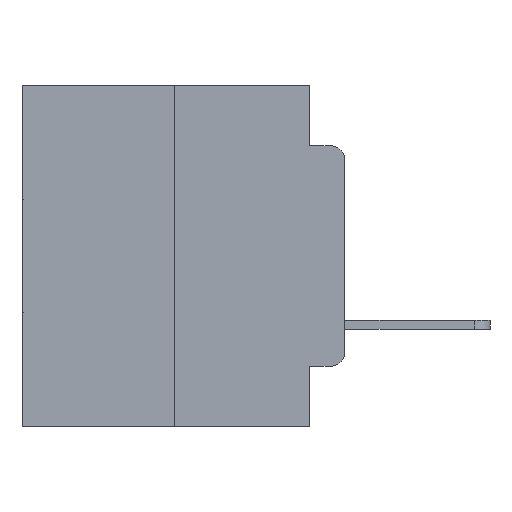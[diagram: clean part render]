
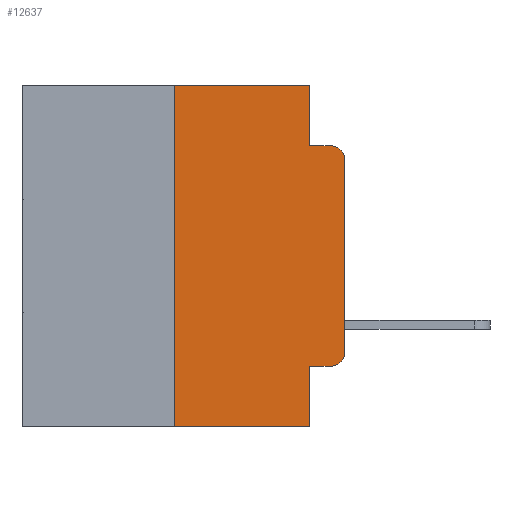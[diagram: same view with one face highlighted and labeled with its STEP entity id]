
A CAD part, left-side view. The second image highlights one B-rep face of the part: STEP entity #12637.
In plain terms, the highlighted planar face has unit normal (-1, 0, 0).
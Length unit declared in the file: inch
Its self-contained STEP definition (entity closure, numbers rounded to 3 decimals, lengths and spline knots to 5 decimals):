
#293 = CARTESIAN_POINT ( 'NONE',  ( 0., 0.473, 0. ) ) ;
#417 = ORIENTED_EDGE ( 'NONE', *, *, #3928, .F. ) ;
#593 = ORIENTED_EDGE ( 'NONE', *, *, #23542, .F. ) ;
#692 = EDGE_CURVE ( 'NONE', #3797, #19112, #18793, .T. ) ;
#924 = ORIENTED_EDGE ( 'NONE', *, *, #692, .F. ) ;
#1023 = ORIENTED_EDGE ( 'NONE', *, *, #10086, .T. ) ;
#1326 = CARTESIAN_POINT ( 'NONE',  ( 0., 0.25, -0.5 ) ) ;
#1830 = ORIENTED_EDGE ( 'NONE', *, *, #25412, .F. ) ;
#2039 = VERTEX_POINT ( 'NONE', #7528 ) ;
#2601 = CIRCLE ( 'NONE', #22563, 0.02 ) ;
#2828 = DIRECTION ( 'NONE',  ( 0., 0., -1. ) ) ;
#2831 = DIRECTION ( 'NONE',  ( -1., 0., 0. ) ) ;
#2906 = CARTESIAN_POINT ( 'NONE',  ( 0., 0.02, -0.1085 ) ) ;
#3025 = LINE ( 'NONE', #20019, #14658 ) ;
#3617 = ORIENTED_EDGE ( 'NONE', *, *, #20435, .T. ) ;
#3686 = VERTEX_POINT ( 'NONE', #26451 ) ;
#3707 = ORIENTED_EDGE ( 'NONE', *, *, #15235, .T. ) ;
#3797 = VERTEX_POINT ( 'NONE', #1326 ) ;
#3928 = EDGE_CURVE ( 'NONE', #12446, #3686, #3025, .T. ) ;
#4108 = VECTOR ( 'NONE', #10217, 39.37008 ) ;
#4351 = EDGE_LOOP ( 'NONE', ( #26457, #26648, #27167, #417, #593, #924, #1023, #1830, #3617, #3707 ) ) ;
#5246 = VERTEX_POINT ( 'NONE', #9247 ) ;
#5438 = LINE ( 'NONE', #25573, #6940 ) ;
#5559 = EDGE_CURVE ( 'NONE', #3686, #22689, #16357, .T. ) ;
#5584 = DIRECTION ( 'NONE',  ( 0., 0., 1. ) ) ;
#6252 = DIRECTION ( 'NONE',  ( 0., 0., 1. ) ) ;
#6285 = CARTESIAN_POINT ( 'NONE',  ( 0., 0.25, 0. ) ) ;
#6411 = DIRECTION ( 'NONE',  ( 0., 0., -1. ) ) ;
#6550 = CARTESIAN_POINT ( 'NONE',  ( 0., 0.051, 0. ) ) ;
#6940 = VECTOR ( 'NONE', #25574, 39.37008 ) ;
#7375 = VECTOR ( 'NONE', #6252, 39.37008 ) ;
#7528 = CARTESIAN_POINT ( 'NONE',  ( 0., 0., -0.3915 ) ) ;
#8077 = VERTEX_POINT ( 'NONE', #16894 ) ;
#8714 = EDGE_CURVE ( 'NONE', #21553, #22689, #25797, .T. ) ;
#9247 = CARTESIAN_POINT ( 'NONE',  ( 0., 0.051, -0.5 ) ) ;
#9537 = DIRECTION ( 'NONE',  ( -1., 0., 0. ) ) ;
#10086 = EDGE_CURVE ( 'NONE', #3797, #5246, #5438, .T. ) ;
#10217 = DIRECTION ( 'NONE',  ( 0., -1., 0. ) ) ;
#10705 = VECTOR ( 'NONE', #22555, 39.37008 ) ;
#11143 = LINE ( 'NONE', #12532, #4108 ) ;
#11466 = CARTESIAN_POINT ( 'NONE',  ( 0., 0.25, 0. ) ) ;
#11860 = CARTESIAN_POINT ( 'NONE',  ( 0., 0.051, -0.4115 ) ) ;
#12024 = LINE ( 'NONE', #16638, #21985 ) ;
#12446 = VERTEX_POINT ( 'NONE', #6550 ) ;
#12532 = CARTESIAN_POINT ( 'NONE',  ( 0., 0.473, 0. ) ) ;
#12637 = ADVANCED_FACE ( 'NONE', ( #23526 ), #18305, .F. ) ;
#12817 = LINE ( 'NONE', #23123, #17580 ) ;
#13178 = CARTESIAN_POINT ( 'NONE',  ( 0., 0.051, -0.4115 ) ) ;
#13281 = EDGE_CURVE ( 'NONE', #2039, #21553, #12024, .T. ) ;
#14658 = VECTOR ( 'NONE', #20696, 39.37008 ) ;
#15235 = EDGE_CURVE ( 'NONE', #8077, #2039, #2601, .T. ) ;
#16220 = VERTEX_POINT ( 'NONE', #13178 ) ;
#16357 = LINE ( 'NONE', #18180, #10705 ) ;
#16638 = CARTESIAN_POINT ( 'NONE',  ( 0., 0., 0. ) ) ;
#16894 = CARTESIAN_POINT ( 'NONE',  ( 0., 0.02, -0.4115 ) ) ;
#17580 = VECTOR ( 'NONE', #6411, 39.37008 ) ;
#18180 = CARTESIAN_POINT ( 'NONE',  ( 0., 0.051, -0.0885 ) ) ;
#18305 = PLANE ( 'NONE',  #24106 ) ;
#18793 = LINE ( 'NONE', #11466, #7375 ) ;
#19045 = CARTESIAN_POINT ( 'NONE',  ( 0., 0., -0.1085 ) ) ;
#19112 = VERTEX_POINT ( 'NONE', #6285 ) ;
#19828 = AXIS2_PLACEMENT_3D ( 'NONE', #2906, #2831, #2828 ) ;
#19989 = DIRECTION ( 'NONE',  ( 0., -1., 0. ) ) ;
#20019 = CARTESIAN_POINT ( 'NONE',  ( 0., 0.051, 0. ) ) ;
#20243 = DIRECTION ( 'NONE',  ( 0., 0., -1. ) ) ;
#20435 = EDGE_CURVE ( 'NONE', #16220, #8077, #26483, .T. ) ;
#20696 = DIRECTION ( 'NONE',  ( 0., 0., -1. ) ) ;
#21553 = VERTEX_POINT ( 'NONE', #19045 ) ;
#21691 = VECTOR ( 'NONE', #19989, 39.37008 ) ;
#21844 = CARTESIAN_POINT ( 'NONE',  ( 0., 0.02, -0.3915 ) ) ;
#21985 = VECTOR ( 'NONE', #5584, 39.37008 ) ;
#22555 = DIRECTION ( 'NONE',  ( 0., -1., 0. ) ) ;
#22563 = AXIS2_PLACEMENT_3D ( 'NONE', #21844, #9537, #23759 ) ;
#22689 = VERTEX_POINT ( 'NONE', #25743 ) ;
#23123 = CARTESIAN_POINT ( 'NONE',  ( 0., 0.051, 0. ) ) ;
#23526 = FACE_OUTER_BOUND ( 'NONE', #4351, .T. ) ;
#23542 = EDGE_CURVE ( 'NONE', #19112, #12446, #11143, .T. ) ;
#23759 = DIRECTION ( 'NONE',  ( 0., 0., -1. ) ) ;
#24106 = AXIS2_PLACEMENT_3D ( 'NONE', #293, #25730, #20243 ) ;
#25412 = EDGE_CURVE ( 'NONE', #16220, #5246, #12817, .T. ) ;
#25573 = CARTESIAN_POINT ( 'NONE',  ( 0., 0.473, -0.5 ) ) ;
#25574 = DIRECTION ( 'NONE',  ( 0., -1., 0. ) ) ;
#25730 = DIRECTION ( 'NONE',  ( 1., 0., 0. ) ) ;
#25743 = CARTESIAN_POINT ( 'NONE',  ( 0., 0.02, -0.0885 ) ) ;
#25797 = CIRCLE ( 'NONE', #19828, 0.02 ) ;
#26451 = CARTESIAN_POINT ( 'NONE',  ( 0., 0.051, -0.0885 ) ) ;
#26457 = ORIENTED_EDGE ( 'NONE', *, *, #13281, .T. ) ;
#26483 = LINE ( 'NONE', #11860, #21691 ) ;
#26648 = ORIENTED_EDGE ( 'NONE', *, *, #8714, .T. ) ;
#27167 = ORIENTED_EDGE ( 'NONE', *, *, #5559, .F. ) ;
